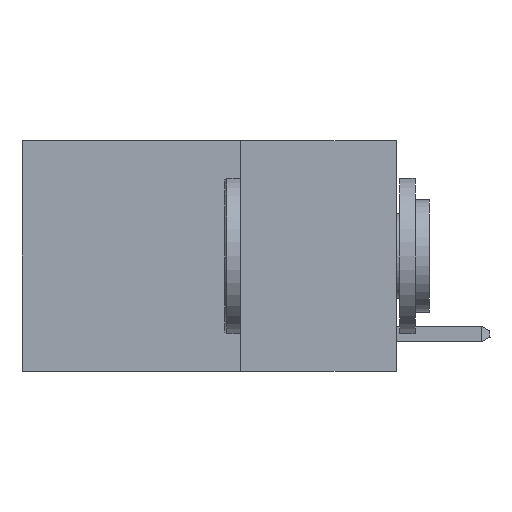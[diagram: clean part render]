
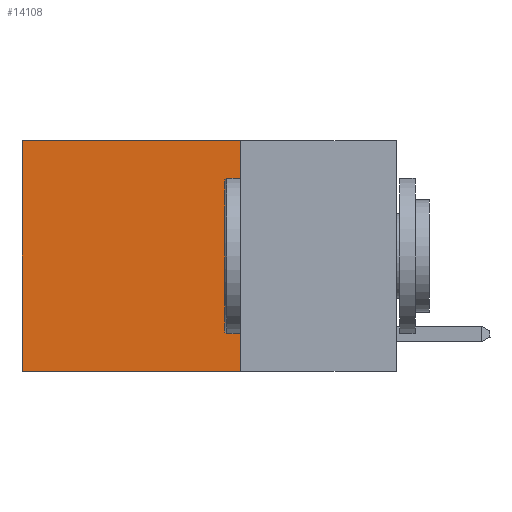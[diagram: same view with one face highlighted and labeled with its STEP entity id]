
A CAD part, left-side view. The second image highlights one B-rep face of the part: STEP entity #14108.
In plain terms, the highlighted planar face has unit normal (-1, 0, 0).
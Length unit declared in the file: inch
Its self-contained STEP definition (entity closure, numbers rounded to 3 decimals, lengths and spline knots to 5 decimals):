
#482 = ORIENTED_EDGE ( 'NONE', *, *, #13414, .T. ) ;
#596 = CARTESIAN_POINT ( 'NONE',  ( 0.2625, 0.6, -0.37 ) ) ;
#3738 = CARTESIAN_POINT ( 'NONE',  ( 0.2625, 0.25, 0. ) ) ;
#3912 = CARTESIAN_POINT ( 'NONE',  ( 0.2625, 0.25, 0. ) ) ;
#4074 = VERTEX_POINT ( 'NONE', #22219 ) ;
#4774 = VERTEX_POINT ( 'NONE', #19418 ) ;
#5702 = CARTESIAN_POINT ( 'NONE',  ( 0.2625, 0.25, 0. ) ) ;
#5824 = FACE_OUTER_BOUND ( 'NONE', #15724, .T. ) ;
#8200 = VERTEX_POINT ( 'NONE', #23993 ) ;
#8867 = CARTESIAN_POINT ( 'NONE',  ( 0.2625, 0.25, -0.37 ) ) ;
#8993 = AXIS2_PLACEMENT_3D ( 'NONE', #3738, #20467, #16997 ) ;
#9090 = VERTEX_POINT ( 'NONE', #596 ) ;
#9223 = LINE ( 'NONE', #8867, #23412 ) ;
#10317 = EDGE_CURVE ( 'NONE', #8200, #9090, #9223, .T. ) ;
#10550 = VECTOR ( 'NONE', #16764, 39.37008 ) ;
#11065 = DIRECTION ( 'NONE',  ( 0., 1., 0. ) ) ;
#11793 = VECTOR ( 'NONE', #18307, 39.37008 ) ;
#12785 = LINE ( 'NONE', #14723, #11793 ) ;
#13193 = LINE ( 'NONE', #5702, #10550 ) ;
#13414 = EDGE_CURVE ( 'NONE', #4074, #9090, #12785, .T. ) ;
#13481 = VECTOR ( 'NONE', #18804, 39.37008 ) ;
#14019 = EDGE_CURVE ( 'NONE', #4774, #4074, #13193, .T. ) ;
#14108 = ADVANCED_FACE ( 'NONE', ( #5824 ), #20823, .F. ) ;
#14723 = CARTESIAN_POINT ( 'NONE',  ( 0.2625, 0.6, 0. ) ) ;
#15724 = EDGE_LOOP ( 'NONE', ( #482, #17691, #22933, #19648 ) ) ;
#16764 = DIRECTION ( 'NONE',  ( 0., 1., 0. ) ) ;
#16997 = DIRECTION ( 'NONE',  ( 0., 0., -1. ) ) ;
#17691 = ORIENTED_EDGE ( 'NONE', *, *, #10317, .F. ) ;
#18307 = DIRECTION ( 'NONE',  ( 0., 0., -1. ) ) ;
#18804 = DIRECTION ( 'NONE',  ( 0., 0., -1. ) ) ;
#19039 = LINE ( 'NONE', #3912, #13481 ) ;
#19418 = CARTESIAN_POINT ( 'NONE',  ( 0.2625, 0.25, 0. ) ) ;
#19648 = ORIENTED_EDGE ( 'NONE', *, *, #14019, .T. ) ;
#20467 = DIRECTION ( 'NONE',  ( 1., 0., 0. ) ) ;
#20823 = PLANE ( 'NONE',  #8993 ) ;
#21741 = EDGE_CURVE ( 'NONE', #4774, #8200, #19039, .T. ) ;
#22219 = CARTESIAN_POINT ( 'NONE',  ( 0.2625, 0.6, 0. ) ) ;
#22933 = ORIENTED_EDGE ( 'NONE', *, *, #21741, .F. ) ;
#23412 = VECTOR ( 'NONE', #11065, 39.37008 ) ;
#23993 = CARTESIAN_POINT ( 'NONE',  ( 0.2625, 0.25, -0.37 ) ) ;
